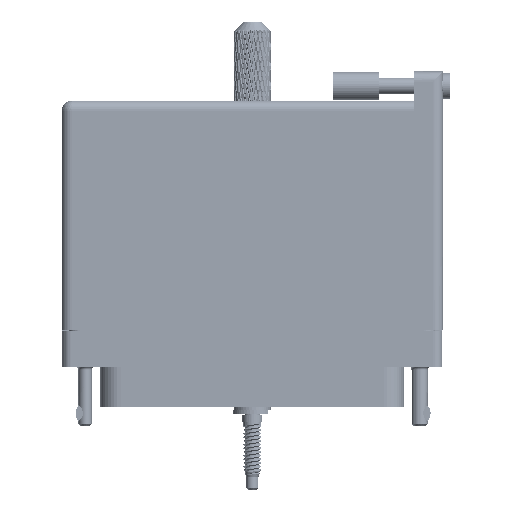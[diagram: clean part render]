
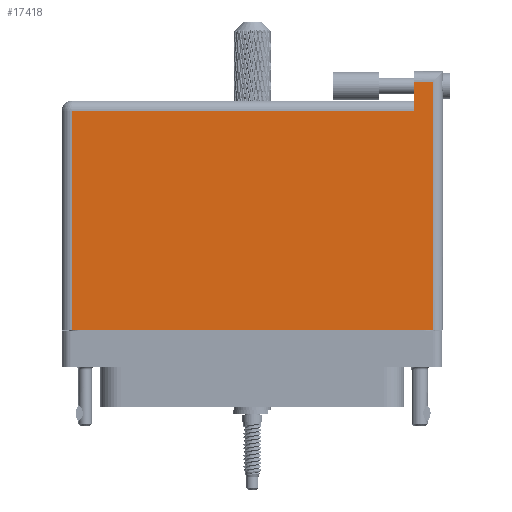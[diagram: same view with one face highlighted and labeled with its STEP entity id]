
A CAD part, front view. The second image highlights one B-rep face of the part: STEP entity #17418.
In plain terms, the highlighted face is planar.
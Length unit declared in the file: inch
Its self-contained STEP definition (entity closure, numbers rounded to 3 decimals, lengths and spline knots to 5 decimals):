
#2342 = EDGE_CURVE ( 'NONE', #73891, #95593, #96661, .T. ) ;
#6300 = VECTOR ( 'NONE', #87740, 39.37008 ) ;
#8473 = LINE ( 'NONE', #77009, #10216 ) ;
#9519 = CARTESIAN_POINT ( 'NONE',  ( 1.103, 1.666, 0.4495 ) ) ;
#10216 = VECTOR ( 'NONE', #20601, 39.37008 ) ;
#10350 = VERTEX_POINT ( 'NONE', #49957 ) ;
#13941 = CARTESIAN_POINT ( 'NONE',  ( -1.3, 1.466, 0.4495 ) ) ;
#17418 = ADVANCED_FACE ( 'NONE', ( #33208 ), #119664, .F. ) ;
#18945 = VECTOR ( 'NONE', #121224, 39.37008 ) ;
#20601 = DIRECTION ( 'NONE',  ( 1., 0., 0. ) ) ;
#22573 = LINE ( 'NONE', #119948, #18945 ) ;
#22944 = ORIENTED_EDGE ( 'NONE', *, *, #64751, .T. ) ;
#24741 = EDGE_CURVE ( 'NONE', #34074, #123565, #81437, .T. ) ;
#25922 = CARTESIAN_POINT ( 'NONE',  ( -1.3, 1.396, 0.4495 ) ) ;
#30305 = EDGE_LOOP ( 'NONE', ( #47830, #76926, #22944, #44817, #126342, #56005 ) ) ;
#32788 = DIRECTION ( 'NONE',  ( 0., 1., 0. ) ) ;
#33208 = FACE_OUTER_BOUND ( 'NONE', #30305, .T. ) ;
#34074 = VERTEX_POINT ( 'NONE', #84503 ) ;
#34735 = VECTOR ( 'NONE', #67217, 39.37008 ) ;
#36624 = VERTEX_POINT ( 'NONE', #104095 ) ;
#36691 = AXIS2_PLACEMENT_3D ( 'NONE', #13941, #92110, #111988 ) ;
#40986 = LINE ( 'NONE', #80036, #6300 ) ;
#44033 = VECTOR ( 'NONE', #32788, 39.37008 ) ;
#44137 = EDGE_CURVE ( 'NONE', #10350, #34074, #8473, .T. ) ;
#44817 = ORIENTED_EDGE ( 'NONE', *, *, #2342, .T. ) ;
#47830 = ORIENTED_EDGE ( 'NONE', *, *, #44137, .T. ) ;
#49957 = CARTESIAN_POINT ( 'NONE',  ( -1.23, -0.1, 0.4495 ) ) ;
#53333 = EDGE_CURVE ( 'NONE', #95593, #36624, #112475, .T. ) ;
#53431 = CARTESIAN_POINT ( 'NONE',  ( 1.23, 1.596, 0.4495 ) ) ;
#56005 = ORIENTED_EDGE ( 'NONE', *, *, #95204, .T. ) ;
#63321 = VECTOR ( 'NONE', #114336, 39.37008 ) ;
#64303 = CARTESIAN_POINT ( 'NONE',  ( 1.103, 1.596, 0.4495 ) ) ;
#64751 = EDGE_CURVE ( 'NONE', #123565, #73891, #40986, .T. ) ;
#67217 = DIRECTION ( 'NONE',  ( 0., -1., 0. ) ) ;
#73891 = VERTEX_POINT ( 'NONE', #64303 ) ;
#76926 = ORIENTED_EDGE ( 'NONE', *, *, #24741, .T. ) ;
#77009 = CARTESIAN_POINT ( 'NONE',  ( -1.3, -0.1, 0.4495 ) ) ;
#80036 = CARTESIAN_POINT ( 'NONE',  ( -1.3, 1.596, 0.4495 ) ) ;
#81437 = LINE ( 'NONE', #120536, #44033 ) ;
#84503 = CARTESIAN_POINT ( 'NONE',  ( 1.23, -0.1, 0.4495 ) ) ;
#87740 = DIRECTION ( 'NONE',  ( -1., 0., 0. ) ) ;
#92110 = DIRECTION ( 'NONE',  ( 0., 0., -1. ) ) ;
#95204 = EDGE_CURVE ( 'NONE', #36624, #10350, #22573, .T. ) ;
#95593 = VERTEX_POINT ( 'NONE', #112745 ) ;
#96661 = LINE ( 'NONE', #9519, #34735 ) ;
#104095 = CARTESIAN_POINT ( 'NONE',  ( -1.23, 1.396, 0.4495 ) ) ;
#111988 = DIRECTION ( 'NONE',  ( -1., 0., 0. ) ) ;
#112475 = LINE ( 'NONE', #25922, #63321 ) ;
#112745 = CARTESIAN_POINT ( 'NONE',  ( 1.103, 1.396, 0.4495 ) ) ;
#114336 = DIRECTION ( 'NONE',  ( -1., 0., 0. ) ) ;
#119664 = PLANE ( 'NONE',  #36691 ) ;
#119948 = CARTESIAN_POINT ( 'NONE',  ( -1.23, -0.1, 0.4495 ) ) ;
#120536 = CARTESIAN_POINT ( 'NONE',  ( 1.23, 1.666, 0.4495 ) ) ;
#121224 = DIRECTION ( 'NONE',  ( 0., -1., 0. ) ) ;
#123565 = VERTEX_POINT ( 'NONE', #53431 ) ;
#126342 = ORIENTED_EDGE ( 'NONE', *, *, #53333, .T. ) ;
